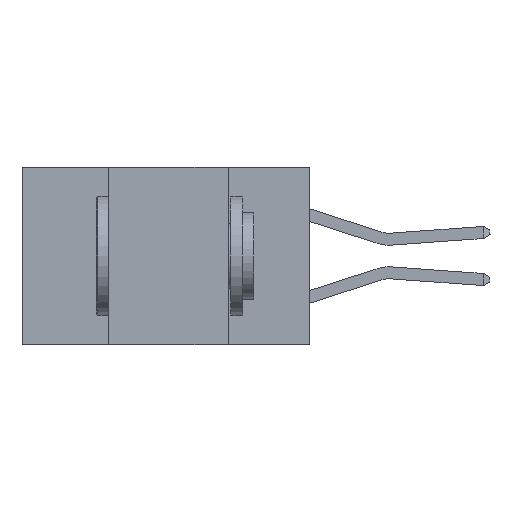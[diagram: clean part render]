
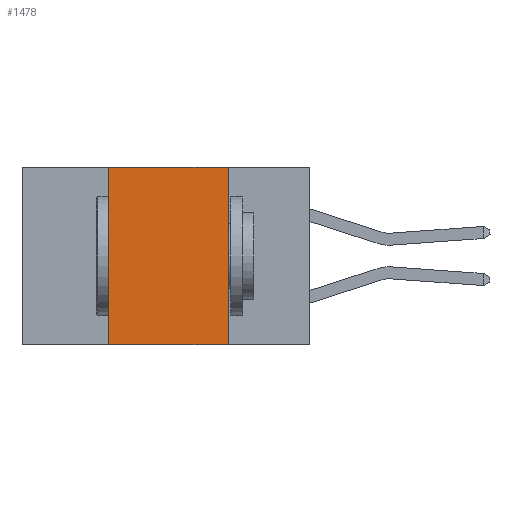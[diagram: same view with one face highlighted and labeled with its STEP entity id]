
A CAD part, left-side view. The second image highlights one B-rep face of the part: STEP entity #1478.
In plain terms, the highlighted planar face has unit normal (-1, 0, 0).
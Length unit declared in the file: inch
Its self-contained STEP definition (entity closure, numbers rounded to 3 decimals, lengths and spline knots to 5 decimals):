
#302 = EDGE_CURVE ( 'NONE', #2146, #4627, #6041, .T. ) ;
#1040 = CARTESIAN_POINT ( 'NONE',  ( 0., 0.17, 0. ) ) ;
#1184 = VERTEX_POINT ( 'NONE', #6543 ) ;
#1274 = EDGE_LOOP ( 'NONE', ( #4261, #7413, #2107, #5429 ) ) ;
#1478 = ADVANCED_FACE ( 'NONE', ( #9176 ), #7417, .F. ) ;
#2107 = ORIENTED_EDGE ( 'NONE', *, *, #11023, .F. ) ;
#2146 = VERTEX_POINT ( 'NONE', #1040 ) ;
#2711 = CARTESIAN_POINT ( 'NONE',  ( 0., 0.6, 0. ) ) ;
#3240 = VECTOR ( 'NONE', #5278, 39.37008 ) ;
#4002 = CARTESIAN_POINT ( 'NONE',  ( 0., 0.42, -0.37 ) ) ;
#4261 = ORIENTED_EDGE ( 'NONE', *, *, #302, .F. ) ;
#4627 = VERTEX_POINT ( 'NONE', #10821 ) ;
#5278 = DIRECTION ( 'NONE',  ( 0., 0., -1. ) ) ;
#5429 = ORIENTED_EDGE ( 'NONE', *, *, #11453, .T. ) ;
#5869 = VECTOR ( 'NONE', #9140, 39.37008 ) ;
#6002 = VECTOR ( 'NONE', #8006, 39.37008 ) ;
#6041 = LINE ( 'NONE', #13423, #3240 ) ;
#6186 = LINE ( 'NONE', #2711, #5869 ) ;
#6394 = VERTEX_POINT ( 'NONE', #4002 ) ;
#6543 = CARTESIAN_POINT ( 'NONE',  ( 0., 0.42, 0. ) ) ;
#7004 = EDGE_CURVE ( 'NONE', #1184, #2146, #6186, .T. ) ;
#7277 = CARTESIAN_POINT ( 'NONE',  ( 0., 0.6, 0. ) ) ;
#7348 = DIRECTION ( 'NONE',  ( 1., 0., 0. ) ) ;
#7413 = ORIENTED_EDGE ( 'NONE', *, *, #7004, .F. ) ;
#7417 = PLANE ( 'NONE',  #13250 ) ;
#7482 = DIRECTION ( 'NONE',  ( 0., 0., -1. ) ) ;
#7822 = VECTOR ( 'NONE', #12708, 39.37008 ) ;
#8006 = DIRECTION ( 'NONE',  ( 0., 0., 1. ) ) ;
#9140 = DIRECTION ( 'NONE',  ( 0., -1., 0. ) ) ;
#9176 = FACE_OUTER_BOUND ( 'NONE', #1274, .T. ) ;
#10573 = LINE ( 'NONE', #11705, #7822 ) ;
#10821 = CARTESIAN_POINT ( 'NONE',  ( 0., 0.17, -0.37 ) ) ;
#10911 = LINE ( 'NONE', #13101, #6002 ) ;
#11023 = EDGE_CURVE ( 'NONE', #6394, #1184, #10911, .T. ) ;
#11453 = EDGE_CURVE ( 'NONE', #6394, #4627, #10573, .T. ) ;
#11705 = CARTESIAN_POINT ( 'NONE',  ( 0., 0.6, -0.37 ) ) ;
#12708 = DIRECTION ( 'NONE',  ( 0., -1., 0. ) ) ;
#13101 = CARTESIAN_POINT ( 'NONE',  ( 0., 0.42, -0.37 ) ) ;
#13250 = AXIS2_PLACEMENT_3D ( 'NONE', #7277, #7348, #7482 ) ;
#13423 = CARTESIAN_POINT ( 'NONE',  ( 0., 0.17, -0.37 ) ) ;
